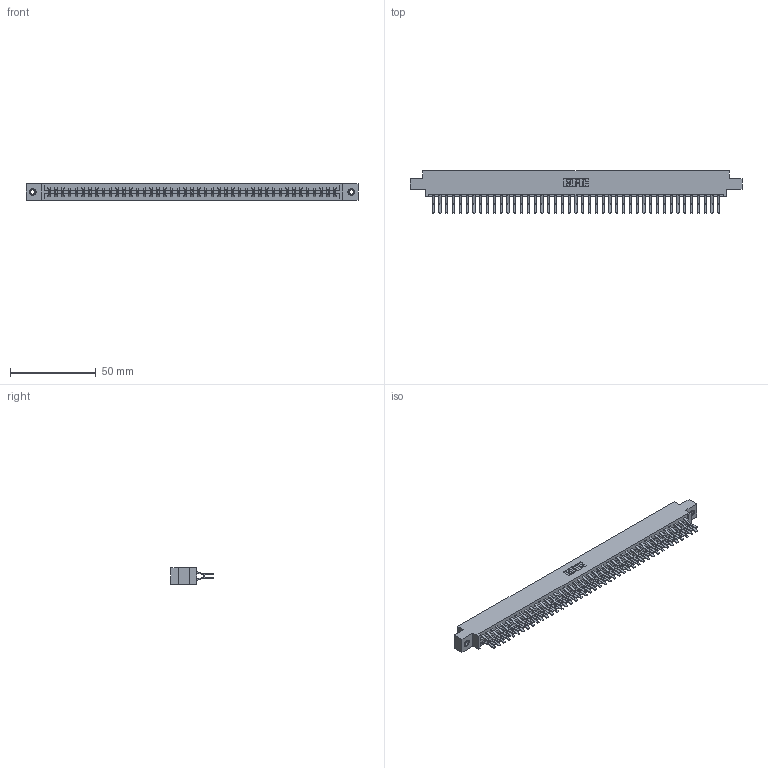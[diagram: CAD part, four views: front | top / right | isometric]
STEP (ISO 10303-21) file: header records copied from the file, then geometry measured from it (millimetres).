
FILE_DESCRIPTION (( 'STEP AP203' ), '1' );
FILE_NAME ('337-086-560-807.STEP', '2018-08-13T02:44:43', ( '' ), ( '' ), 'SwSTEP 2.0', 'SolidWorks 2016', '' );
FILE_SCHEMA (( 'CONFIG_CONTROL_DESIGN' ));
Length unit declared in the file: inch
Products named in the file (4): 337 Part_0.170 Offset - 0.156 Dia-TI; 345-292-001_560 Tail; 345-250-001_345-250-005-103; 337-086-560-807
Assembly tree (89 placements, depth 2):
  337-086-560-807
    337 Part_0.170 Offset - 0.156 Dia-TI
    345-292-001_560 Tail  x86
    345-250-001_345-250-005-103  x2
Bounding box: 193.4 x 24.78 x 9.4 mm (x, y, z)
Volume: 20827.5 mm3; surface area: 25330.5 mm2
Topology: 89 solids, 89 shells, 4994 faces, 14821 edges, 9758 vertices
Faces by surface type: plane 3374, cylinder 1604, cone 12, torus 4
Entity records: 34616 total; most frequent: CARTESIAN_POINT 5813, ORIENTED_EDGE 5742, DIRECTION 4977, EDGE_CURVE 2871, VECTOR 2719, LINE 2719, VERTEX_POINT 1908, AXIS2_PLACEMENT_3D 1129
